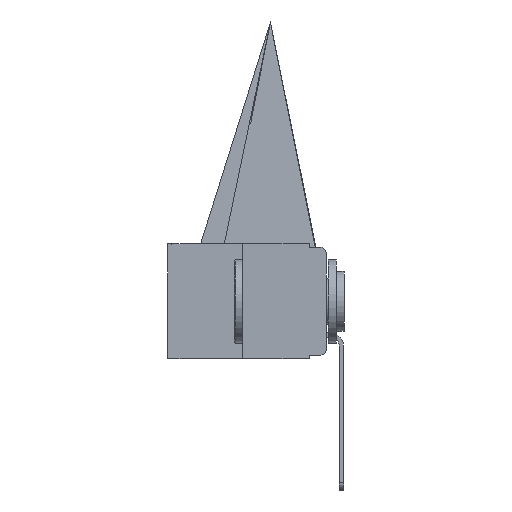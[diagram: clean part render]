
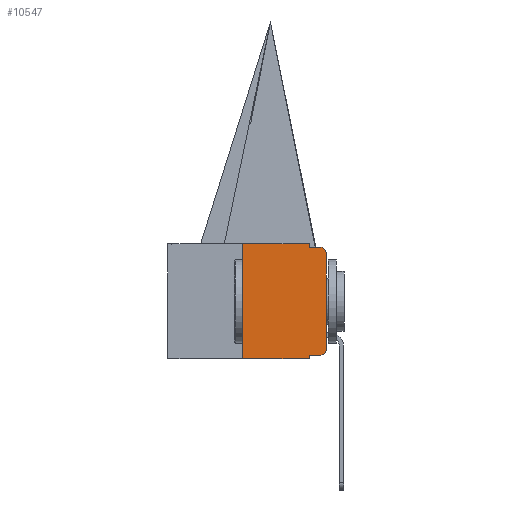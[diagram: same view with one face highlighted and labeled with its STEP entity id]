
A CAD part, left-side view. The second image highlights one B-rep face of the part: STEP entity #10547.
In plain terms, the highlighted planar face has unit normal (-1, 0, 0).
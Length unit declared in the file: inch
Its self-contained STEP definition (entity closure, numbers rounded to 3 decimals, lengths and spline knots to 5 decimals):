
#141 = CARTESIAN_POINT ( 'NONE',  ( 0., 0.25, 0. ) ) ;
#926 = VECTOR ( 'NONE', #2870, 39.37008 ) ;
#1009 = ORIENTED_EDGE ( 'NONE', *, *, #11391, .T. ) ;
#1118 = VERTEX_POINT ( 'NONE', #15507 ) ;
#1536 = ORIENTED_EDGE ( 'NONE', *, *, #3341, .T. ) ;
#2202 = EDGE_CURVE ( 'NONE', #7271, #1118, #14741, .T. ) ;
#2213 = CARTESIAN_POINT ( 'NONE',  ( 0., 0.051, -0.333 ) ) ;
#2458 = LINE ( 'NONE', #2213, #6772 ) ;
#2852 = VERTEX_POINT ( 'NONE', #10029 ) ;
#2870 = DIRECTION ( 'NONE',  ( 0., 0., -1. ) ) ;
#3341 = EDGE_CURVE ( 'NONE', #14264, #7271, #2458, .T. ) ;
#3447 = CARTESIAN_POINT ( 'NONE',  ( 0., 0.051, -0.333 ) ) ;
#3640 = CARTESIAN_POINT ( 'NONE',  ( 0., 0.02, -0.313 ) ) ;
#3701 = VECTOR ( 'NONE', #6867, 39.37008 ) ;
#4105 = CARTESIAN_POINT ( 'NONE',  ( 0., 0.473, 0. ) ) ;
#4359 = CARTESIAN_POINT ( 'NONE',  ( 0., 0.25, 0. ) ) ;
#4380 = VECTOR ( 'NONE', #7530, 39.37008 ) ;
#4414 = EDGE_CURVE ( 'NONE', #14264, #2852, #12516, .T. ) ;
#4562 = VECTOR ( 'NONE', #18509, 39.37008 ) ;
#4913 = ORIENTED_EDGE ( 'NONE', *, *, #5546, .F. ) ;
#5521 = AXIS2_PLACEMENT_3D ( 'NONE', #3640, #11199, #14978 ) ;
#5546 = EDGE_CURVE ( 'NONE', #13319, #16035, #8557, .T. ) ;
#5601 = CIRCLE ( 'NONE', #20128, 0.02 ) ;
#5711 = EDGE_CURVE ( 'NONE', #16035, #11187, #13378, .T. ) ;
#5793 = CARTESIAN_POINT ( 'NONE',  ( 0., 0.051, -0.01 ) ) ;
#5829 = EDGE_LOOP ( 'NONE', ( #6667, #11278, #15283, #16205, #20200, #4913, #1009, #17632, #1536, #10051 ) ) ;
#6534 = VECTOR ( 'NONE', #11890, 39.37008 ) ;
#6584 = EDGE_CURVE ( 'NONE', #11187, #14745, #14071, .T. ) ;
#6608 = DIRECTION ( 'NONE',  ( -1., 0., 0. ) ) ;
#6667 = ORIENTED_EDGE ( 'NONE', *, *, #9671, .T. ) ;
#6714 = AXIS2_PLACEMENT_3D ( 'NONE', #4105, #16494, #7353 ) ;
#6772 = VECTOR ( 'NONE', #14733, 39.37008 ) ;
#6867 = DIRECTION ( 'NONE',  ( 0., 0., -1. ) ) ;
#7271 = VERTEX_POINT ( 'NONE', #16376 ) ;
#7272 = CARTESIAN_POINT ( 'NONE',  ( 0., 0.473, -0.343 ) ) ;
#7353 = DIRECTION ( 'NONE',  ( 0., 0., -1. ) ) ;
#7530 = DIRECTION ( 'NONE',  ( 0., 0., 1. ) ) ;
#7586 = EDGE_CURVE ( 'NONE', #14745, #10789, #20329, .T. ) ;
#7832 = CARTESIAN_POINT ( 'NONE',  ( 0., 0.051, -0.01 ) ) ;
#7931 = DIRECTION ( 'NONE',  ( 0., -1., 0. ) ) ;
#8557 = LINE ( 'NONE', #4359, #4380 ) ;
#8626 = EDGE_CURVE ( 'NONE', #19910, #10789, #5601, .T. ) ;
#9671 = EDGE_CURVE ( 'NONE', #1118, #19910, #11614, .T. ) ;
#10029 = CARTESIAN_POINT ( 'NONE',  ( 0., 0.051, -0.343 ) ) ;
#10051 = ORIENTED_EDGE ( 'NONE', *, *, #2202, .T. ) ;
#10259 = VECTOR ( 'NONE', #7931, 39.37008 ) ;
#10547 = ADVANCED_FACE ( 'NONE', ( #10594 ), #14998, .F. ) ;
#10594 = FACE_OUTER_BOUND ( 'NONE', #5829, .T. ) ;
#10789 = VERTEX_POINT ( 'NONE', #17568 ) ;
#11122 = VECTOR ( 'NONE', #15743, 39.37008 ) ;
#11187 = VERTEX_POINT ( 'NONE', #15765 ) ;
#11199 = DIRECTION ( 'NONE',  ( -1., 0., 0. ) ) ;
#11278 = ORIENTED_EDGE ( 'NONE', *, *, #8626, .T. ) ;
#11391 = EDGE_CURVE ( 'NONE', #13319, #2852, #17155, .T. ) ;
#11539 = CARTESIAN_POINT ( 'NONE',  ( 0., 0.051, 0. ) ) ;
#11614 = LINE ( 'NONE', #20210, #11122 ) ;
#11890 = DIRECTION ( 'NONE',  ( 0., -1., 0. ) ) ;
#12516 = LINE ( 'NONE', #11539, #3701 ) ;
#13319 = VERTEX_POINT ( 'NONE', #14956 ) ;
#13378 = LINE ( 'NONE', #15551, #10259 ) ;
#14071 = LINE ( 'NONE', #18196, #926 ) ;
#14264 = VERTEX_POINT ( 'NONE', #3447 ) ;
#14733 = DIRECTION ( 'NONE',  ( 0., -1., 0. ) ) ;
#14741 = CIRCLE ( 'NONE', #5521, 0.02 ) ;
#14745 = VERTEX_POINT ( 'NONE', #5793 ) ;
#14956 = CARTESIAN_POINT ( 'NONE',  ( 0., 0.25, -0.343 ) ) ;
#14978 = DIRECTION ( 'NONE',  ( 0., 0., -1. ) ) ;
#14998 = PLANE ( 'NONE',  #6714 ) ;
#15283 = ORIENTED_EDGE ( 'NONE', *, *, #7586, .F. ) ;
#15507 = CARTESIAN_POINT ( 'NONE',  ( 0., 0., -0.313 ) ) ;
#15551 = CARTESIAN_POINT ( 'NONE',  ( 0., 0.473, 0. ) ) ;
#15742 = CARTESIAN_POINT ( 'NONE',  ( 0., 0.02, -0.03 ) ) ;
#15743 = DIRECTION ( 'NONE',  ( 0., 0., 1. ) ) ;
#15765 = CARTESIAN_POINT ( 'NONE',  ( 0., 0.051, 0. ) ) ;
#16035 = VERTEX_POINT ( 'NONE', #141 ) ;
#16205 = ORIENTED_EDGE ( 'NONE', *, *, #6584, .F. ) ;
#16376 = CARTESIAN_POINT ( 'NONE',  ( 0., 0.02, -0.333 ) ) ;
#16494 = DIRECTION ( 'NONE',  ( 1., 0., 0. ) ) ;
#16963 = CARTESIAN_POINT ( 'NONE',  ( 0., 0., -0.03 ) ) ;
#17155 = LINE ( 'NONE', #7272, #6534 ) ;
#17245 = DIRECTION ( 'NONE',  ( 0., 0., -1. ) ) ;
#17568 = CARTESIAN_POINT ( 'NONE',  ( 0., 0.02, -0.01 ) ) ;
#17632 = ORIENTED_EDGE ( 'NONE', *, *, #4414, .F. ) ;
#18196 = CARTESIAN_POINT ( 'NONE',  ( 0., 0.051, 0. ) ) ;
#18509 = DIRECTION ( 'NONE',  ( 0., -1., 0. ) ) ;
#19910 = VERTEX_POINT ( 'NONE', #16963 ) ;
#20128 = AXIS2_PLACEMENT_3D ( 'NONE', #15742, #6608, #17245 ) ;
#20200 = ORIENTED_EDGE ( 'NONE', *, *, #5711, .F. ) ;
#20210 = CARTESIAN_POINT ( 'NONE',  ( 0., 0., 0. ) ) ;
#20329 = LINE ( 'NONE', #7832, #4562 ) ;
